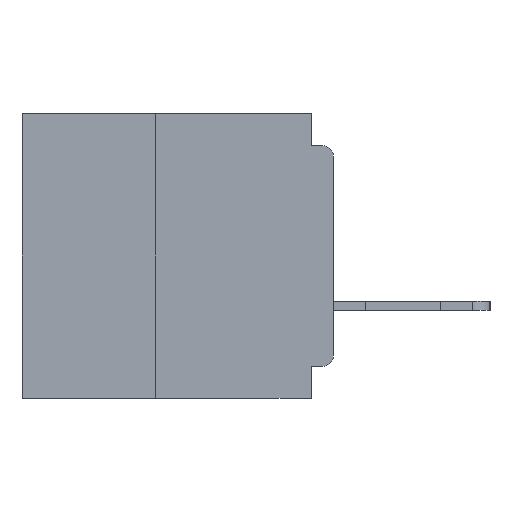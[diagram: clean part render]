
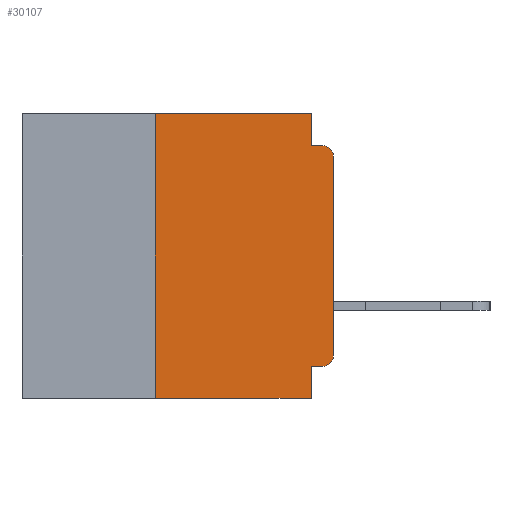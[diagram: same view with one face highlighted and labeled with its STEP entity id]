
A CAD part, left-side view. The second image highlights one B-rep face of the part: STEP entity #30107.
In plain terms, the highlighted planar face has unit normal (-1, 0, 0).
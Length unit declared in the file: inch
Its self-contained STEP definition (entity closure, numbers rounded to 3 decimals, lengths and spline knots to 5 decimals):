
#234 = DIRECTION ( 'NONE',  ( 0., 0., -1. ) ) ;
#378 = CIRCLE ( 'NONE', #15255, 0.015 ) ;
#800 = EDGE_CURVE ( 'NONE', #10756, #20043, #11646, .T. ) ;
#1487 = VECTOR ( 'NONE', #16053, 39.37008 ) ;
#2818 = ORIENTED_EDGE ( 'NONE', *, *, #16859, .F. ) ;
#2864 = ORIENTED_EDGE ( 'NONE', *, *, #46499, .F. ) ;
#4378 = DIRECTION ( 'NONE',  ( 0., -1., 0. ) ) ;
#4818 = CARTESIAN_POINT ( 'NONE',  ( 0., 0., -0.34 ) ) ;
#6189 = VERTEX_POINT ( 'NONE', #40047 ) ;
#6381 = VERTEX_POINT ( 'NONE', #21678 ) ;
#7249 = VERTEX_POINT ( 'NONE', #15533 ) ;
#8455 = LINE ( 'NONE', #29750, #16358 ) ;
#8907 = DIRECTION ( 'NONE',  ( 1., 0., 0. ) ) ;
#9068 = CARTESIAN_POINT ( 'NONE',  ( 0., 0.25, -0.4 ) ) ;
#9536 = CARTESIAN_POINT ( 'NONE',  ( 0., 0.015, -0.355 ) ) ;
#10068 = CARTESIAN_POINT ( 'NONE',  ( 0., 0.25, -0.4 ) ) ;
#10256 = EDGE_CURVE ( 'NONE', #6381, #10756, #38773, .T. ) ;
#10743 = DIRECTION ( 'NONE',  ( 0., 1., 0. ) ) ;
#10756 = VERTEX_POINT ( 'NONE', #44202 ) ;
#10973 = VECTOR ( 'NONE', #10743, 39.37008 ) ;
#11530 = CARTESIAN_POINT ( 'NONE',  ( 0., 0.031, -0.045 ) ) ;
#11646 = LINE ( 'NONE', #26716, #20660 ) ;
#12143 = CARTESIAN_POINT ( 'NONE',  ( 0., 0.437, -0.4 ) ) ;
#12189 = CARTESIAN_POINT ( 'NONE',  ( 0., 0., -0.045 ) ) ;
#12671 = ORIENTED_EDGE ( 'NONE', *, *, #10256, .F. ) ;
#13169 = DIRECTION ( 'NONE',  ( 0., 0., 1. ) ) ;
#14875 = VERTEX_POINT ( 'NONE', #10068 ) ;
#15255 = AXIS2_PLACEMENT_3D ( 'NONE', #45509, #22144, #49447 ) ;
#15533 = CARTESIAN_POINT ( 'NONE',  ( 0., 0.031, -0.4 ) ) ;
#16053 = DIRECTION ( 'NONE',  ( 0., -1., 0. ) ) ;
#16149 = VECTOR ( 'NONE', #13169, 39.37008 ) ;
#16358 = VECTOR ( 'NONE', #21963, 39.37008 ) ;
#16859 = EDGE_CURVE ( 'NONE', #20043, #37060, #32503, .T. ) ;
#17114 = LINE ( 'NONE', #23982, #36509 ) ;
#18081 = AXIS2_PLACEMENT_3D ( 'NONE', #46892, #23510, #234 ) ;
#18863 = LINE ( 'NONE', #12143, #37044 ) ;
#19347 = VECTOR ( 'NONE', #20922, 39.37008 ) ;
#20043 = VERTEX_POINT ( 'NONE', #11530 ) ;
#20660 = VECTOR ( 'NONE', #26624, 39.37008 ) ;
#20922 = DIRECTION ( 'NONE',  ( 0., -1., 0. ) ) ;
#21325 = ORIENTED_EDGE ( 'NONE', *, *, #45533, .T. ) ;
#21678 = CARTESIAN_POINT ( 'NONE',  ( 0., 0.25, 0. ) ) ;
#21774 = CARTESIAN_POINT ( 'NONE',  ( 0., 0.437, 0. ) ) ;
#21963 = DIRECTION ( 'NONE',  ( 0., 0., -1. ) ) ;
#22144 = DIRECTION ( 'NONE',  ( -1., 0., 0. ) ) ;
#23510 = DIRECTION ( 'NONE',  ( -1., 0., 0. ) ) ;
#23765 = ORIENTED_EDGE ( 'NONE', *, *, #41211, .T. ) ;
#23982 = CARTESIAN_POINT ( 'NONE',  ( 0., 0., 0. ) ) ;
#24193 = VERTEX_POINT ( 'NONE', #4818 ) ;
#24872 = CARTESIAN_POINT ( 'NONE',  ( 0., 0.015, -0.045 ) ) ;
#25567 = EDGE_CURVE ( 'NONE', #39083, #24193, #378, .T. ) ;
#26313 = CIRCLE ( 'NONE', #18081, 0.015 ) ;
#26423 = LINE ( 'NONE', #9068, #16149 ) ;
#26624 = DIRECTION ( 'NONE',  ( 0., 0., -1. ) ) ;
#26716 = CARTESIAN_POINT ( 'NONE',  ( 0., 0.031, 0. ) ) ;
#27165 = ORIENTED_EDGE ( 'NONE', *, *, #25567, .T. ) ;
#27498 = EDGE_LOOP ( 'NONE', ( #21325, #23765, #2818, #38696, #12671, #27781, #48542, #31438, #2864, #27165 ) ) ;
#27781 = ORIENTED_EDGE ( 'NONE', *, *, #48752, .F. ) ;
#27908 = DIRECTION ( 'NONE',  ( 0., 0., 1. ) ) ;
#29695 = AXIS2_PLACEMENT_3D ( 'NONE', #39762, #8907, #36026 ) ;
#29750 = CARTESIAN_POINT ( 'NONE',  ( 0., 0.031, -0.4 ) ) ;
#30107 = ADVANCED_FACE ( 'NONE', ( #31119 ), #32133, .F. ) ;
#31119 = FACE_OUTER_BOUND ( 'NONE', #27498, .T. ) ;
#31438 = ORIENTED_EDGE ( 'NONE', *, *, #33032, .F. ) ;
#32133 = PLANE ( 'NONE',  #29695 ) ;
#32503 = LINE ( 'NONE', #12189, #1487 ) ;
#33032 = EDGE_CURVE ( 'NONE', #6189, #7249, #8455, .T. ) ;
#33943 = CARTESIAN_POINT ( 'NONE',  ( 0., 0., -0.355 ) ) ;
#34171 = VERTEX_POINT ( 'NONE', #40577 ) ;
#36026 = DIRECTION ( 'NONE',  ( 0., 0., -1. ) ) ;
#36509 = VECTOR ( 'NONE', #27908, 39.37008 ) ;
#37044 = VECTOR ( 'NONE', #4378, 39.37008 ) ;
#37060 = VERTEX_POINT ( 'NONE', #24872 ) ;
#38696 = ORIENTED_EDGE ( 'NONE', *, *, #800, .F. ) ;
#38773 = LINE ( 'NONE', #21774, #19347 ) ;
#39083 = VERTEX_POINT ( 'NONE', #9536 ) ;
#39762 = CARTESIAN_POINT ( 'NONE',  ( 0., 0.437, 0. ) ) ;
#40047 = CARTESIAN_POINT ( 'NONE',  ( 0., 0.031, -0.355 ) ) ;
#40577 = CARTESIAN_POINT ( 'NONE',  ( 0., 0., -0.06 ) ) ;
#40646 = LINE ( 'NONE', #33943, #10973 ) ;
#41211 = EDGE_CURVE ( 'NONE', #34171, #37060, #26313, .T. ) ;
#44202 = CARTESIAN_POINT ( 'NONE',  ( 0., 0.031, 0. ) ) ;
#45509 = CARTESIAN_POINT ( 'NONE',  ( 0., 0.015, -0.34 ) ) ;
#45533 = EDGE_CURVE ( 'NONE', #24193, #34171, #17114, .T. ) ;
#46127 = EDGE_CURVE ( 'NONE', #14875, #7249, #18863, .T. ) ;
#46499 = EDGE_CURVE ( 'NONE', #39083, #6189, #40646, .T. ) ;
#46892 = CARTESIAN_POINT ( 'NONE',  ( 0., 0.015, -0.06 ) ) ;
#48542 = ORIENTED_EDGE ( 'NONE', *, *, #46127, .T. ) ;
#48752 = EDGE_CURVE ( 'NONE', #14875, #6381, #26423, .T. ) ;
#49447 = DIRECTION ( 'NONE',  ( 0., 0., -1. ) ) ;
